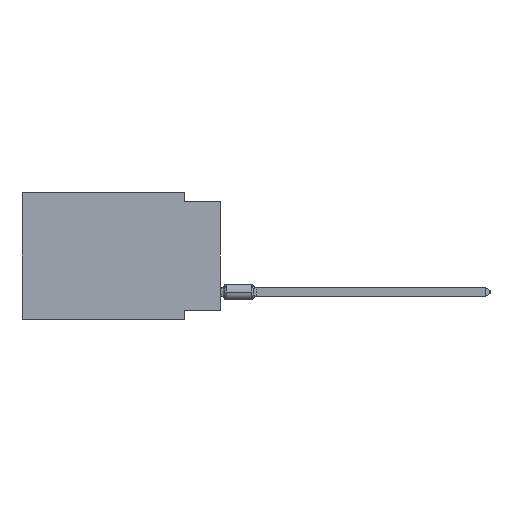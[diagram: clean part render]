
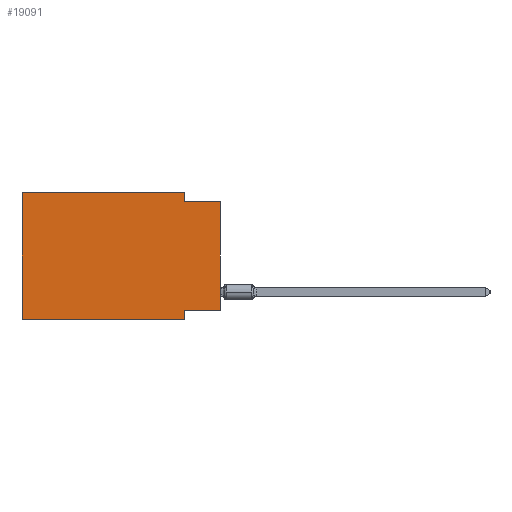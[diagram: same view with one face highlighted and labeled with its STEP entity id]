
A CAD part, left-side view. The second image highlights one B-rep face of the part: STEP entity #19091.
In plain terms, the highlighted planar face has unit normal (-1, 0, 0).
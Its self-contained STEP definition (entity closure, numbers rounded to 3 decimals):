
#464 = VECTOR ( 'NONE', #5450, 1000. ) ;
#586 = VERTEX_POINT ( 'NONE', #8603 ) ;
#708 = CARTESIAN_POINT ( 'NONE',  ( 0., 13.97, 0. ) ) ;
#781 = LINE ( 'NONE', #11740, #12928 ) ;
#1246 = ORIENTED_EDGE ( 'NONE', *, *, #6874, .F. ) ;
#1387 = FACE_OUTER_BOUND ( 'NONE', #13807, .T. ) ;
#1621 = EDGE_CURVE ( 'NONE', #19901, #22633, #28670, .T. ) ;
#2254 = CARTESIAN_POINT ( 'NONE',  ( 0., 2.54, -8.255 ) ) ;
#2330 = CARTESIAN_POINT ( 'NONE',  ( 0., 2.54, 0. ) ) ;
#3222 = DIRECTION ( 'NONE',  ( 0., 0., -1. ) ) ;
#3671 = VECTOR ( 'NONE', #18856, 1000. ) ;
#4486 = ORIENTED_EDGE ( 'NONE', *, *, #6031, .F. ) ;
#4521 = VERTEX_POINT ( 'NONE', #8942 ) ;
#4538 = DIRECTION ( 'NONE',  ( 0., -1., 0. ) ) ;
#4822 = LINE ( 'NONE', #9797, #11562 ) ;
#5450 = DIRECTION ( 'NONE',  ( 0., 1., 0. ) ) ;
#6031 = EDGE_CURVE ( 'NONE', #13170, #13629, #12283, .T. ) ;
#6754 = CARTESIAN_POINT ( 'NONE',  ( 0., 13.97, 0. ) ) ;
#6874 = EDGE_CURVE ( 'NONE', #4521, #13170, #20937, .T. ) ;
#7773 = CARTESIAN_POINT ( 'NONE',  ( 0., 2.54, -8.89 ) ) ;
#7814 = CARTESIAN_POINT ( 'NONE',  ( 0., 0., -8.255 ) ) ;
#8340 = ORIENTED_EDGE ( 'NONE', *, *, #16077, .T. ) ;
#8603 = CARTESIAN_POINT ( 'NONE',  ( 0., 2.54, -0.635 ) ) ;
#8942 = CARTESIAN_POINT ( 'NONE',  ( 0., 0., -8.255 ) ) ;
#9481 = ORIENTED_EDGE ( 'NONE', *, *, #13357, .F. ) ;
#9797 = CARTESIAN_POINT ( 'NONE',  ( 0., 13.97, -8.89 ) ) ;
#9965 = CARTESIAN_POINT ( 'NONE',  ( 0., 0., -0.635 ) ) ;
#10297 = DIRECTION ( 'NONE',  ( 1., 0., 0. ) ) ;
#10765 = ORIENTED_EDGE ( 'NONE', *, *, #12456, .F. ) ;
#10898 = DIRECTION ( 'NONE',  ( 0., 0., 1. ) ) ;
#11560 = CARTESIAN_POINT ( 'NONE',  ( 0., 2.54, -8.89 ) ) ;
#11562 = VECTOR ( 'NONE', #18690, 1000. ) ;
#11685 = EDGE_CURVE ( 'NONE', #20512, #19901, #781, .T. ) ;
#11740 = CARTESIAN_POINT ( 'NONE',  ( 0., 13.97, 0. ) ) ;
#12123 = EDGE_CURVE ( 'NONE', #20512, #13629, #4822, .T. ) ;
#12198 = VECTOR ( 'NONE', #10898, 1000. ) ;
#12283 = LINE ( 'NONE', #7773, #17732 ) ;
#12456 = EDGE_CURVE ( 'NONE', #22633, #586, #22212, .T. ) ;
#12928 = VECTOR ( 'NONE', #14482, 1000. ) ;
#13135 = DIRECTION ( 'NONE',  ( 0., 0., -1. ) ) ;
#13170 = VERTEX_POINT ( 'NONE', #2254 ) ;
#13207 = CARTESIAN_POINT ( 'NONE',  ( 0., 13.97, -8.89 ) ) ;
#13357 = EDGE_CURVE ( 'NONE', #586, #22124, #21063, .T. ) ;
#13629 = VERTEX_POINT ( 'NONE', #11560 ) ;
#13807 = EDGE_LOOP ( 'NONE', ( #8340, #9481, #10765, #16377, #21085, #27414, #4486, #1246 ) ) ;
#14482 = DIRECTION ( 'NONE',  ( 0., 0., 1. ) ) ;
#14810 = PLANE ( 'NONE',  #23564 ) ;
#16077 = EDGE_CURVE ( 'NONE', #4521, #22124, #28865, .T. ) ;
#16377 = ORIENTED_EDGE ( 'NONE', *, *, #1621, .F. ) ;
#17000 = DIRECTION ( 'NONE',  ( 0., 0., -1. ) ) ;
#17732 = VECTOR ( 'NONE', #3222, 1000. ) ;
#17737 = CARTESIAN_POINT ( 'NONE',  ( 0., 0., 0. ) ) ;
#18690 = DIRECTION ( 'NONE',  ( 0., -1., 0. ) ) ;
#18856 = DIRECTION ( 'NONE',  ( 0., -1., 0. ) ) ;
#19091 = ADVANCED_FACE ( 'NONE', ( #1387 ), #14810, .F. ) ;
#19479 = VECTOR ( 'NONE', #13135, 1000. ) ;
#19901 = VERTEX_POINT ( 'NONE', #708 ) ;
#20512 = VERTEX_POINT ( 'NONE', #13207 ) ;
#20730 = VECTOR ( 'NONE', #4538, 1000. ) ;
#20937 = LINE ( 'NONE', #7814, #464 ) ;
#21063 = LINE ( 'NONE', #9965, #3671 ) ;
#21085 = ORIENTED_EDGE ( 'NONE', *, *, #11685, .F. ) ;
#22124 = VERTEX_POINT ( 'NONE', #26546 ) ;
#22212 = LINE ( 'NONE', #2330, #19479 ) ;
#22633 = VERTEX_POINT ( 'NONE', #26646 ) ;
#23564 = AXIS2_PLACEMENT_3D ( 'NONE', #25506, #10297, #17000 ) ;
#25506 = CARTESIAN_POINT ( 'NONE',  ( 0., 13.97, 0. ) ) ;
#26546 = CARTESIAN_POINT ( 'NONE',  ( 0., 0., -0.635 ) ) ;
#26646 = CARTESIAN_POINT ( 'NONE',  ( 0., 2.54, 0. ) ) ;
#27414 = ORIENTED_EDGE ( 'NONE', *, *, #12123, .T. ) ;
#28670 = LINE ( 'NONE', #6754, #20730 ) ;
#28865 = LINE ( 'NONE', #17737, #12198 ) ;
